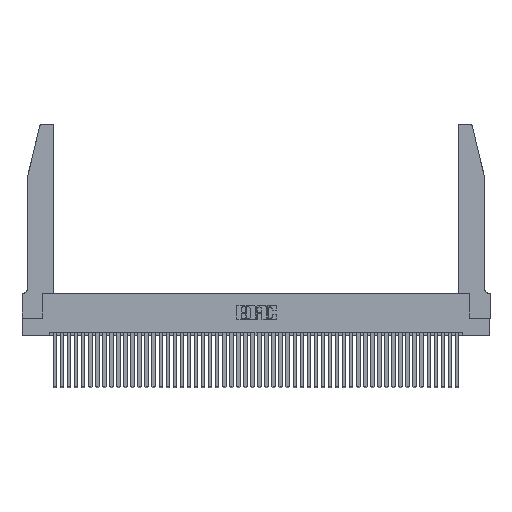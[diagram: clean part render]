
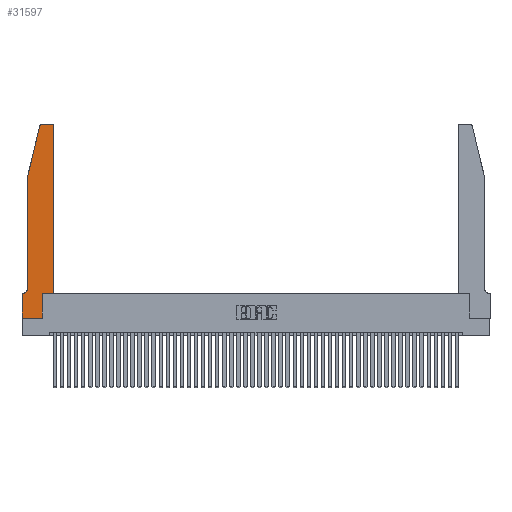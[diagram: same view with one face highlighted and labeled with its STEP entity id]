
A CAD part, top view. The second image highlights one B-rep face of the part: STEP entity #31597.
In plain terms, the highlighted planar face has unit normal (0, 0, 1).
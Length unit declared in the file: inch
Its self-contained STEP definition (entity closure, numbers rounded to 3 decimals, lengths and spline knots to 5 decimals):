
#693 = EDGE_CURVE ( 'NONE', #17927, #14973, #33016, .T. ) ;
#937 = ORIENTED_EDGE ( 'NONE', *, *, #20766, .T. ) ;
#1194 = AXIS2_PLACEMENT_3D ( 'NONE', #7606, #33488, #11354 ) ;
#2799 = DIRECTION ( 'NONE',  ( -1., 0., 0. ) ) ;
#3447 = DIRECTION ( 'NONE',  ( 0., 0., 1. ) ) ;
#4273 = DIRECTION ( 'NONE',  ( 0., 0., 1. ) ) ;
#4563 = VERTEX_POINT ( 'NONE', #31904 ) ;
#4685 = DIRECTION ( 'NONE',  ( 0., -1., 0. ) ) ;
#5269 = VERTEX_POINT ( 'NONE', #33245 ) ;
#5533 = EDGE_CURVE ( 'NONE', #21073, #19645, #32076, .T. ) ;
#5699 = CARTESIAN_POINT ( 'NONE',  ( 0.4505, 0.35, 0.37 ) ) ;
#6173 = LINE ( 'NONE', #19972, #14873 ) ;
#6900 = LINE ( 'NONE', #8557, #25436 ) ;
#7432 = AXIS2_PLACEMENT_3D ( 'NONE', #10881, #3447, #29406 ) ;
#7606 = CARTESIAN_POINT ( 'NONE',  ( 0.284, 2.72, 0.37 ) ) ;
#7937 = VERTEX_POINT ( 'NONE', #31186 ) ;
#8223 = VECTOR ( 'NONE', #2799, 39.37008 ) ;
#8557 = CARTESIAN_POINT ( 'NONE',  ( 0.4505, 0.35, 0.37 ) ) ;
#9519 = CARTESIAN_POINT ( 'NONE',  ( 0.0755, 2., 0.37 ) ) ;
#10379 = CARTESIAN_POINT ( 'NONE',  ( 0.0755, 0.42, 0.37 ) ) ;
#10881 = CARTESIAN_POINT ( 'NONE',  ( 0., 0.35, 0.37 ) ) ;
#10993 = LINE ( 'NONE', #9519, #39214 ) ;
#11354 = DIRECTION ( 'NONE',  ( 1., 0., 0. ) ) ;
#11877 = ORIENTED_EDGE ( 'NONE', *, *, #5533, .T. ) ;
#11912 = EDGE_CURVE ( 'NONE', #5269, #17927, #14721, .T. ) ;
#12114 = EDGE_CURVE ( 'NONE', #4563, #39050, #6173, .T. ) ;
#12290 = VERTEX_POINT ( 'NONE', #17199 ) ;
#12663 = CARTESIAN_POINT ( 'NONE',  ( 0.0055, 0.42, 0.37 ) ) ;
#14721 = CIRCLE ( 'NONE', #17957, 0.03 ) ;
#14774 = ORIENTED_EDGE ( 'NONE', *, *, #12114, .T. ) ;
#14873 = VECTOR ( 'NONE', #38303, 39.37008 ) ;
#14909 = CARTESIAN_POINT ( 'NONE',  ( 0., 0.35, 0.37 ) ) ;
#14973 = VERTEX_POINT ( 'NONE', #27017 ) ;
#16385 = DIRECTION ( 'NONE',  ( -1., 0., 0. ) ) ;
#17030 = EDGE_LOOP ( 'NONE', ( #42471, #34795, #937, #44378, #11877, #28295, #33102, #14774, #42497, #20182, #38286, #41316 ) ) ;
#17199 = CARTESIAN_POINT ( 'NONE',  ( 0.2865, 0.35, 0.37 ) ) ;
#17288 = EDGE_CURVE ( 'NONE', #14973, #18449, #36935, .T. ) ;
#17360 = FACE_OUTER_BOUND ( 'NONE', #17030, .T. ) ;
#17927 = VERTEX_POINT ( 'NONE', #44917 ) ;
#17957 = AXIS2_PLACEMENT_3D ( 'NONE', #26504, #4273, #30215 ) ;
#18449 = VERTEX_POINT ( 'NONE', #36857 ) ;
#19158 = LINE ( 'NONE', #43331, #37580 ) ;
#19645 = VERTEX_POINT ( 'NONE', #43334 ) ;
#19653 = AXIS2_PLACEMENT_3D ( 'NONE', #12663, #38444, #16385 ) ;
#19972 = CARTESIAN_POINT ( 'NONE',  ( 0., 0., 0.37 ) ) ;
#20182 = ORIENTED_EDGE ( 'NONE', *, *, #31849, .T. ) ;
#20766 = EDGE_CURVE ( 'NONE', #18449, #7937, #23206, .T. ) ;
#21073 = VERTEX_POINT ( 'NONE', #10379 ) ;
#21386 = CARTESIAN_POINT ( 'NONE',  ( 0.0755, 0.35, 0.37 ) ) ;
#23206 = LINE ( 'NONE', #46627, #31873 ) ;
#25436 = VECTOR ( 'NONE', #37889, 39.37008 ) ;
#26504 = CARTESIAN_POINT ( 'NONE',  ( 0.4205, 2.72, 0.37 ) ) ;
#26584 = LINE ( 'NONE', #41529, #34092 ) ;
#27017 = CARTESIAN_POINT ( 'NONE',  ( 0.284, 2.75, 0.37 ) ) ;
#28295 = ORIENTED_EDGE ( 'NONE', *, *, #40886, .T. ) ;
#29044 = VERTEX_POINT ( 'NONE', #5699 ) ;
#29245 = PLANE ( 'NONE',  #7432 ) ;
#29378 = EDGE_CURVE ( 'NONE', #39050, #12290, #45405, .T. ) ;
#29406 = DIRECTION ( 'NONE',  ( 1., 0., 0. ) ) ;
#30215 = DIRECTION ( 'NONE',  ( 1., 0., 0. ) ) ;
#31186 = CARTESIAN_POINT ( 'NONE',  ( 0.0755, 2., 0.37 ) ) ;
#31597 = ADVANCED_FACE ( 'NONE', ( #17360 ), #29245, .T. ) ;
#31841 = VECTOR ( 'NONE', #41975, 39.37008 ) ;
#31849 = EDGE_CURVE ( 'NONE', #12290, #29044, #6900, .T. ) ;
#31873 = VECTOR ( 'NONE', #35710, 39.37008 ) ;
#31904 = CARTESIAN_POINT ( 'NONE',  ( 0., 0., 0.37 ) ) ;
#31985 = EDGE_CURVE ( 'NONE', #7937, #21073, #10993, .T. ) ;
#32076 = CIRCLE ( 'NONE', #19653, 0.07 ) ;
#33016 = LINE ( 'NONE', #45675, #31841 ) ;
#33102 = ORIENTED_EDGE ( 'NONE', *, *, #42345, .T. ) ;
#33245 = CARTESIAN_POINT ( 'NONE',  ( 0.4505, 2.72, 0.37 ) ) ;
#33488 = DIRECTION ( 'NONE',  ( 0., 0., 1. ) ) ;
#34092 = VECTOR ( 'NONE', #4685, 39.37008 ) ;
#34795 = ORIENTED_EDGE ( 'NONE', *, *, #17288, .T. ) ;
#35710 = DIRECTION ( 'NONE',  ( -0.239, -0.971, 0. ) ) ;
#36809 = VECTOR ( 'NONE', #37483, 39.37008 ) ;
#36857 = CARTESIAN_POINT ( 'NONE',  ( 0.25487, 2.72718, 0.37 ) ) ;
#36935 = CIRCLE ( 'NONE', #1194, 0.03 ) ;
#37483 = DIRECTION ( 'NONE',  ( 0., 1., 0. ) ) ;
#37580 = VECTOR ( 'NONE', #39643, 39.37008 ) ;
#37638 = LINE ( 'NONE', #21386, #8223 ) ;
#37875 = VERTEX_POINT ( 'NONE', #14909 ) ;
#37889 = DIRECTION ( 'NONE',  ( 1., 0., 0. ) ) ;
#38286 = ORIENTED_EDGE ( 'NONE', *, *, #44873, .T. ) ;
#38303 = DIRECTION ( 'NONE',  ( 1., 0., 0. ) ) ;
#38444 = DIRECTION ( 'NONE',  ( 0., 0., -1. ) ) ;
#39050 = VERTEX_POINT ( 'NONE', #43561 ) ;
#39214 = VECTOR ( 'NONE', #42511, 39.37008 ) ;
#39643 = DIRECTION ( 'NONE',  ( 0., 1., 0. ) ) ;
#40886 = EDGE_CURVE ( 'NONE', #19645, #37875, #37638, .T. ) ;
#41316 = ORIENTED_EDGE ( 'NONE', *, *, #11912, .T. ) ;
#41529 = CARTESIAN_POINT ( 'NONE',  ( 0., 0., 0.37 ) ) ;
#41975 = DIRECTION ( 'NONE',  ( -1., 0., 0. ) ) ;
#42345 = EDGE_CURVE ( 'NONE', #37875, #4563, #26584, .T. ) ;
#42471 = ORIENTED_EDGE ( 'NONE', *, *, #693, .T. ) ;
#42497 = ORIENTED_EDGE ( 'NONE', *, *, #29378, .T. ) ;
#42511 = DIRECTION ( 'NONE',  ( 0., -1., 0. ) ) ;
#43331 = CARTESIAN_POINT ( 'NONE',  ( 0.4505, 0.35, 0.37 ) ) ;
#43334 = CARTESIAN_POINT ( 'NONE',  ( 0.0055, 0.35, 0.37 ) ) ;
#43561 = CARTESIAN_POINT ( 'NONE',  ( 0.2865, 0., 0.37 ) ) ;
#44378 = ORIENTED_EDGE ( 'NONE', *, *, #31985, .T. ) ;
#44867 = CARTESIAN_POINT ( 'NONE',  ( 0.2865, 0.35, 0.37 ) ) ;
#44873 = EDGE_CURVE ( 'NONE', #29044, #5269, #19158, .T. ) ;
#44917 = CARTESIAN_POINT ( 'NONE',  ( 0.4205, 2.75, 0.37 ) ) ;
#45405 = LINE ( 'NONE', #44867, #36809 ) ;
#45675 = CARTESIAN_POINT ( 'NONE',  ( 0.2605, 2.75, 0.37 ) ) ;
#46627 = CARTESIAN_POINT ( 'NONE',  ( 0.0755, 2., 0.37 ) ) ;
